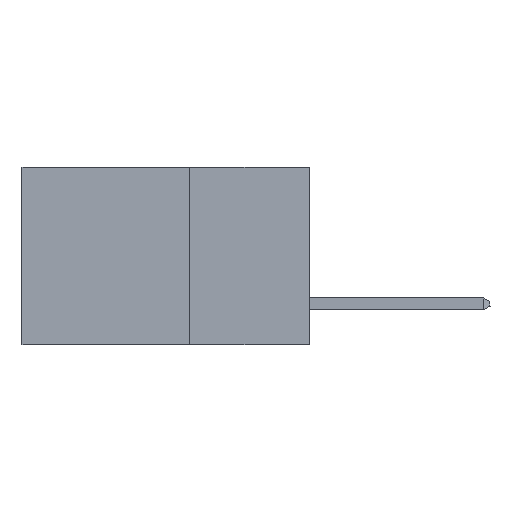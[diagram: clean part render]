
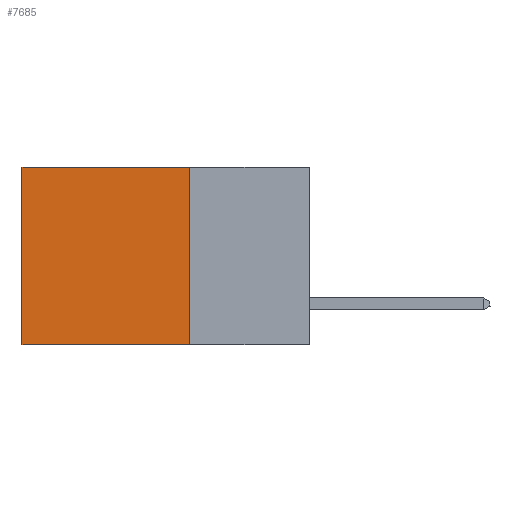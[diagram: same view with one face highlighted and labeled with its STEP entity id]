
A CAD part, left-side view. The second image highlights one B-rep face of the part: STEP entity #7685.
In plain terms, the highlighted planar face has unit normal (-1, 0, 0).
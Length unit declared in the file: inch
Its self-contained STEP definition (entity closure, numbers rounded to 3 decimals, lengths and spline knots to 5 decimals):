
#237 = FACE_OUTER_BOUND ( 'NONE', #13944, .T. ) ;
#688 = EDGE_CURVE ( 'NONE', #33043, #26857, #10427, .T. ) ;
#1438 = EDGE_CURVE ( 'NONE', #36759, #33043, #35501, .T. ) ;
#1610 = ORIENTED_EDGE ( 'NONE', *, *, #15190, .T. ) ;
#3676 = VECTOR ( 'NONE', #6348, 39.37008 ) ;
#3779 = VECTOR ( 'NONE', #14934, 39.37008 ) ;
#6167 = LINE ( 'NONE', #20921, #15118 ) ;
#6348 = DIRECTION ( 'NONE',  ( 0., 1., 0. ) ) ;
#6522 = EDGE_CURVE ( 'NONE', #10624, #26857, #6167, .T. ) ;
#7685 = ADVANCED_FACE ( 'NONE', ( #237 ), #15115, .F. ) ;
#9126 = CARTESIAN_POINT ( 'NONE',  ( 0.2875, 0.25, -0.37 ) ) ;
#10427 = LINE ( 'NONE', #9126, #3676 ) ;
#10624 = VERTEX_POINT ( 'NONE', #31884 ) ;
#13205 = ORIENTED_EDGE ( 'NONE', *, *, #688, .F. ) ;
#13944 = EDGE_LOOP ( 'NONE', ( #14460, #13205, #15091, #1610 ) ) ;
#14460 = ORIENTED_EDGE ( 'NONE', *, *, #6522, .T. ) ;
#14934 = DIRECTION ( 'NONE',  ( 0., 1., 0. ) ) ;
#15091 = ORIENTED_EDGE ( 'NONE', *, *, #1438, .F. ) ;
#15115 = PLANE ( 'NONE',  #17277 ) ;
#15118 = VECTOR ( 'NONE', #23810, 39.37008 ) ;
#15190 = EDGE_CURVE ( 'NONE', #36759, #10624, #29319, .T. ) ;
#17277 = AXIS2_PLACEMENT_3D ( 'NONE', #35435, #20763, #18009 ) ;
#18009 = DIRECTION ( 'NONE',  ( 0., 0., -1. ) ) ;
#20587 = CARTESIAN_POINT ( 'NONE',  ( 0.2875, 0.25, 0. ) ) ;
#20763 = DIRECTION ( 'NONE',  ( 1., 0., 0. ) ) ;
#20921 = CARTESIAN_POINT ( 'NONE',  ( 0.2875, 0.6, 0. ) ) ;
#23578 = CARTESIAN_POINT ( 'NONE',  ( 0.2875, 0.25, -0.37 ) ) ;
#23810 = DIRECTION ( 'NONE',  ( 0., 0., -1. ) ) ;
#23853 = CARTESIAN_POINT ( 'NONE',  ( 0.2875, 0.25, 0. ) ) ;
#26857 = VERTEX_POINT ( 'NONE', #36511 ) ;
#27388 = CARTESIAN_POINT ( 'NONE',  ( 0.2875, 0.25, 0. ) ) ;
#27892 = VECTOR ( 'NONE', #33937, 39.37008 ) ;
#29319 = LINE ( 'NONE', #20587, #3779 ) ;
#31884 = CARTESIAN_POINT ( 'NONE',  ( 0.2875, 0.6, 0. ) ) ;
#33043 = VERTEX_POINT ( 'NONE', #23578 ) ;
#33937 = DIRECTION ( 'NONE',  ( 0., 0., -1. ) ) ;
#35435 = CARTESIAN_POINT ( 'NONE',  ( 0.2875, 0.25, 0. ) ) ;
#35501 = LINE ( 'NONE', #27388, #27892 ) ;
#36511 = CARTESIAN_POINT ( 'NONE',  ( 0.2875, 0.6, -0.37 ) ) ;
#36759 = VERTEX_POINT ( 'NONE', #23853 ) ;
